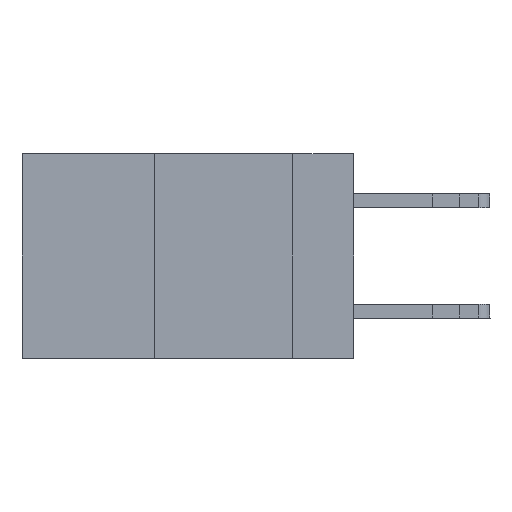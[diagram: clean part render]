
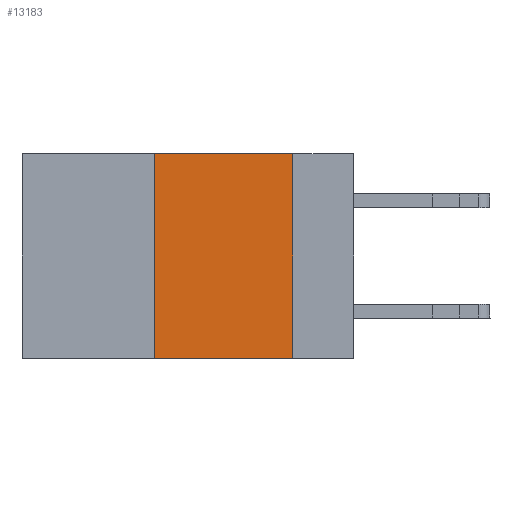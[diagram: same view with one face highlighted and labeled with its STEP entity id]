
A CAD part, left-side view. The second image highlights one B-rep face of the part: STEP entity #13183.
In plain terms, the highlighted planar face has unit normal (-1, 0, 0).
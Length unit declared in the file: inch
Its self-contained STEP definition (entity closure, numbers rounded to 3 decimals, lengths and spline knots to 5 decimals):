
#951 = CARTESIAN_POINT ( 'NONE',  ( 0., 0.36, 0. ) ) ;
#1185 = LINE ( 'NONE', #8773, #6259 ) ;
#1515 = FACE_OUTER_BOUND ( 'NONE', #13077, .T. ) ;
#1859 = DIRECTION ( 'NONE',  ( 0., 0., -1. ) ) ;
#2078 = PLANE ( 'NONE',  #17015 ) ;
#2828 = CARTESIAN_POINT ( 'NONE',  ( 0., 0.36, -0.37 ) ) ;
#3391 = DIRECTION ( 'NONE',  ( 0., -1., 0. ) ) ;
#3695 = VERTEX_POINT ( 'NONE', #10880 ) ;
#4044 = DIRECTION ( 'NONE',  ( 0., 0., -1. ) ) ;
#6259 = VECTOR ( 'NONE', #21832, 39.37008 ) ;
#7114 = CARTESIAN_POINT ( 'NONE',  ( 0., 0.6, -0.37 ) ) ;
#8773 = CARTESIAN_POINT ( 'NONE',  ( 0., 0.36, 0. ) ) ;
#10880 = CARTESIAN_POINT ( 'NONE',  ( 0., 0.11, -0.37 ) ) ;
#13077 = EDGE_LOOP ( 'NONE', ( #14327, #17334, #20063, #20372 ) ) ;
#13081 = VECTOR ( 'NONE', #24097, 39.37008 ) ;
#13183 = ADVANCED_FACE ( 'NONE', ( #1515 ), #2078, .F. ) ;
#14096 = VERTEX_POINT ( 'NONE', #2828 ) ;
#14281 = LINE ( 'NONE', #22258, #13081 ) ;
#14327 = ORIENTED_EDGE ( 'NONE', *, *, #16475, .F. ) ;
#14542 = VECTOR ( 'NONE', #3391, 39.37008 ) ;
#15132 = LINE ( 'NONE', #7114, #14542 ) ;
#15247 = DIRECTION ( 'NONE',  ( 1., 0., 0. ) ) ;
#16409 = LINE ( 'NONE', #18752, #21886 ) ;
#16475 = EDGE_CURVE ( 'NONE', #18813, #3695, #16409, .T. ) ;
#17015 = AXIS2_PLACEMENT_3D ( 'NONE', #18865, #15247, #4044 ) ;
#17334 = ORIENTED_EDGE ( 'NONE', *, *, #21958, .F. ) ;
#17483 = VERTEX_POINT ( 'NONE', #951 ) ;
#18492 = CARTESIAN_POINT ( 'NONE',  ( 0., 0.11, 0. ) ) ;
#18752 = CARTESIAN_POINT ( 'NONE',  ( 0., 0.11, 0. ) ) ;
#18813 = VERTEX_POINT ( 'NONE', #18492 ) ;
#18865 = CARTESIAN_POINT ( 'NONE',  ( 0., 0.6, 0. ) ) ;
#20063 = ORIENTED_EDGE ( 'NONE', *, *, #23748, .F. ) ;
#20372 = ORIENTED_EDGE ( 'NONE', *, *, #22517, .T. ) ;
#21832 = DIRECTION ( 'NONE',  ( 0., 0., 1. ) ) ;
#21886 = VECTOR ( 'NONE', #1859, 39.37008 ) ;
#21958 = EDGE_CURVE ( 'NONE', #17483, #18813, #14281, .T. ) ;
#22258 = CARTESIAN_POINT ( 'NONE',  ( 0., 0.6, 0. ) ) ;
#22517 = EDGE_CURVE ( 'NONE', #14096, #3695, #15132, .T. ) ;
#23748 = EDGE_CURVE ( 'NONE', #14096, #17483, #1185, .T. ) ;
#24097 = DIRECTION ( 'NONE',  ( 0., -1., 0. ) ) ;
